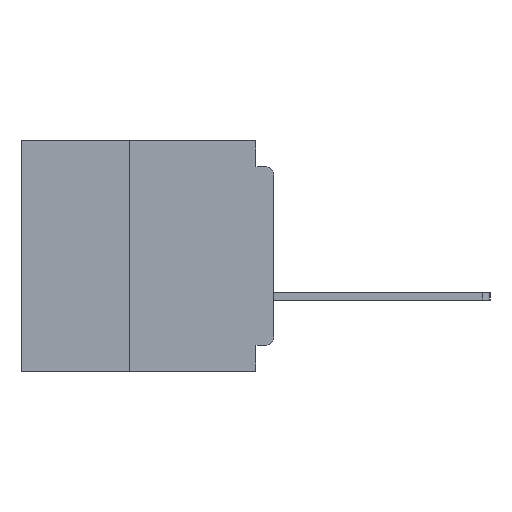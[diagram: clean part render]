
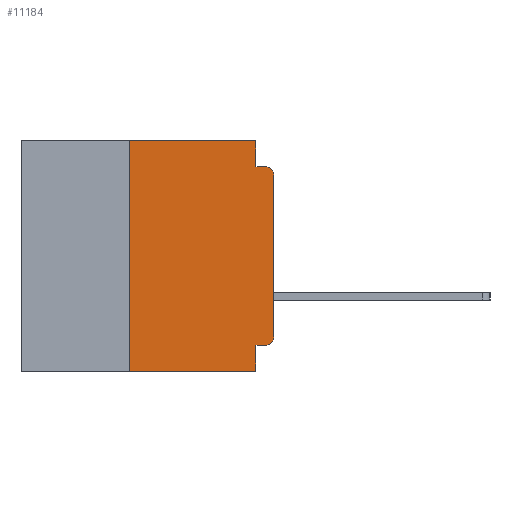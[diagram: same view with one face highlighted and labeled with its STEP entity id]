
A CAD part, left-side view. The second image highlights one B-rep face of the part: STEP entity #11184.
In plain terms, the highlighted planar face has unit normal (-1, 0, 0).
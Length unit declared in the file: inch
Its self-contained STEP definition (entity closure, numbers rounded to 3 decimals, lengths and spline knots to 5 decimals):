
#19 = VERTEX_POINT ( 'NONE', #27709 ) ;
#135 = DIRECTION ( 'NONE',  ( 0., 0., -1. ) ) ;
#626 = ORIENTED_EDGE ( 'NONE', *, *, #46272, .T. ) ;
#731 = EDGE_CURVE ( 'NONE', #19723, #12528, #26812, .T. ) ;
#824 = VERTEX_POINT ( 'NONE', #867 ) ;
#867 = CARTESIAN_POINT ( 'NONE',  ( 0., 0.015, -0.355 ) ) ;
#1844 = ORIENTED_EDGE ( 'NONE', *, *, #19192, .F. ) ;
#2385 = DIRECTION ( 'NONE',  ( 0., 0., 1. ) ) ;
#2674 = CARTESIAN_POINT ( 'NONE',  ( 0., 0.437, 0. ) ) ;
#3344 = VECTOR ( 'NONE', #25679, 39.37008 ) ;
#3861 = CARTESIAN_POINT ( 'NONE',  ( 0., 0.031, 0. ) ) ;
#3969 = ORIENTED_EDGE ( 'NONE', *, *, #53702, .F. ) ;
#4319 = LINE ( 'NONE', #39994, #36277 ) ;
#5255 = ORIENTED_EDGE ( 'NONE', *, *, #39785, .T. ) ;
#5553 = VECTOR ( 'NONE', #36344, 39.37008 ) ;
#6567 = VECTOR ( 'NONE', #48807, 39.37008 ) ;
#10461 = VECTOR ( 'NONE', #47812, 39.37008 ) ;
#10559 = FACE_OUTER_BOUND ( 'NONE', #38248, .T. ) ;
#11108 = DIRECTION ( 'NONE',  ( 0., 0., -1. ) ) ;
#11184 = ADVANCED_FACE ( 'NONE', ( #10559 ), #27646, .F. ) ;
#11774 = LINE ( 'NONE', #43641, #10461 ) ;
#12528 = VERTEX_POINT ( 'NONE', #16664 ) ;
#13629 = CIRCLE ( 'NONE', #18632, 0.015 ) ;
#13636 = CARTESIAN_POINT ( 'NONE',  ( 0., 0.031, -0.045 ) ) ;
#13940 = DIRECTION ( 'NONE',  ( -1., 0., 0. ) ) ;
#14809 = EDGE_CURVE ( 'NONE', #824, #19, #47758, .T. ) ;
#14965 = LINE ( 'NONE', #25106, #27288 ) ;
#15482 = CARTESIAN_POINT ( 'NONE',  ( 0., 0.437, -0.4 ) ) ;
#16664 = CARTESIAN_POINT ( 'NONE',  ( 0., 0.015, -0.045 ) ) ;
#17048 = ORIENTED_EDGE ( 'NONE', *, *, #33296, .F. ) ;
#17088 = VECTOR ( 'NONE', #29060, 39.37008 ) ;
#17284 = CARTESIAN_POINT ( 'NONE',  ( 0., 0.25, 0. ) ) ;
#17345 = AXIS2_PLACEMENT_3D ( 'NONE', #2674, #36056, #11108 ) ;
#17492 = LINE ( 'NONE', #37198, #38333 ) ;
#18632 = AXIS2_PLACEMENT_3D ( 'NONE', #38877, #13940, #43110 ) ;
#19192 = EDGE_CURVE ( 'NONE', #30142, #20017, #14965, .T. ) ;
#19723 = VERTEX_POINT ( 'NONE', #24155 ) ;
#20017 = VERTEX_POINT ( 'NONE', #13636 ) ;
#22823 = ORIENTED_EDGE ( 'NONE', *, *, #731, .T. ) ;
#23717 = CARTESIAN_POINT ( 'NONE',  ( 0., 0., 0. ) ) ;
#24155 = CARTESIAN_POINT ( 'NONE',  ( 0., 0., -0.06 ) ) ;
#24227 = DIRECTION ( 'NONE',  ( 0., 0., -1. ) ) ;
#24740 = DIRECTION ( 'NONE',  ( 0., -1., 0. ) ) ;
#25106 = CARTESIAN_POINT ( 'NONE',  ( 0., 0.031, 0. ) ) ;
#25481 = LINE ( 'NONE', #53989, #17088 ) ;
#25487 = ORIENTED_EDGE ( 'NONE', *, *, #44854, .T. ) ;
#25679 = DIRECTION ( 'NONE',  ( 0., 1., 0. ) ) ;
#26812 = CIRCLE ( 'NONE', #31151, 0.015 ) ;
#27288 = VECTOR ( 'NONE', #135, 39.37008 ) ;
#27646 = PLANE ( 'NONE',  #17345 ) ;
#27709 = CARTESIAN_POINT ( 'NONE',  ( 0., 0.031, -0.355 ) ) ;
#28604 = EDGE_CURVE ( 'NONE', #19, #39397, #11774, .T. ) ;
#28773 = LINE ( 'NONE', #15482, #6567 ) ;
#28944 = CARTESIAN_POINT ( 'NONE',  ( 0., 0.015, -0.06 ) ) ;
#29060 = DIRECTION ( 'NONE',  ( 0., -1., 0. ) ) ;
#29624 = VERTEX_POINT ( 'NONE', #17284 ) ;
#29932 = CARTESIAN_POINT ( 'NONE',  ( 0., 0., -0.355 ) ) ;
#30142 = VERTEX_POINT ( 'NONE', #3861 ) ;
#31151 = AXIS2_PLACEMENT_3D ( 'NONE', #28944, #34149, #24227 ) ;
#32635 = CARTESIAN_POINT ( 'NONE',  ( 0., 0., -0.34 ) ) ;
#33296 = EDGE_CURVE ( 'NONE', #20017, #12528, #25481, .T. ) ;
#33319 = ORIENTED_EDGE ( 'NONE', *, *, #45220, .F. ) ;
#34149 = DIRECTION ( 'NONE',  ( -1., 0., 0. ) ) ;
#36056 = DIRECTION ( 'NONE',  ( 1., 0., 0. ) ) ;
#36277 = VECTOR ( 'NONE', #2385, 39.37008 ) ;
#36344 = DIRECTION ( 'NONE',  ( 0., 0., 1. ) ) ;
#37198 = CARTESIAN_POINT ( 'NONE',  ( 0., 0.437, 0. ) ) ;
#38161 = CARTESIAN_POINT ( 'NONE',  ( 0., 0.25, -0.4 ) ) ;
#38248 = EDGE_LOOP ( 'NONE', ( #626, #22823, #17048, #1844, #33319, #3969, #5255, #41217, #42534, #25487 ) ) ;
#38333 = VECTOR ( 'NONE', #24740, 39.37008 ) ;
#38877 = CARTESIAN_POINT ( 'NONE',  ( 0., 0.015, -0.34 ) ) ;
#39397 = VERTEX_POINT ( 'NONE', #50464 ) ;
#39785 = EDGE_CURVE ( 'NONE', #44751, #39397, #28773, .T. ) ;
#39994 = CARTESIAN_POINT ( 'NONE',  ( 0., 0.25, -0.4 ) ) ;
#41217 = ORIENTED_EDGE ( 'NONE', *, *, #28604, .F. ) ;
#42534 = ORIENTED_EDGE ( 'NONE', *, *, #14809, .F. ) ;
#42936 = VERTEX_POINT ( 'NONE', #32635 ) ;
#43110 = DIRECTION ( 'NONE',  ( 0., 0., -1. ) ) ;
#43641 = CARTESIAN_POINT ( 'NONE',  ( 0., 0.031, -0.4 ) ) ;
#44751 = VERTEX_POINT ( 'NONE', #38161 ) ;
#44854 = EDGE_CURVE ( 'NONE', #824, #42936, #13629, .T. ) ;
#45220 = EDGE_CURVE ( 'NONE', #29624, #30142, #17492, .T. ) ;
#46272 = EDGE_CURVE ( 'NONE', #42936, #19723, #49938, .T. ) ;
#47758 = LINE ( 'NONE', #29932, #3344 ) ;
#47812 = DIRECTION ( 'NONE',  ( 0., 0., -1. ) ) ;
#48807 = DIRECTION ( 'NONE',  ( 0., -1., 0. ) ) ;
#49938 = LINE ( 'NONE', #23717, #5553 ) ;
#50464 = CARTESIAN_POINT ( 'NONE',  ( 0., 0.031, -0.4 ) ) ;
#53702 = EDGE_CURVE ( 'NONE', #44751, #29624, #4319, .T. ) ;
#53989 = CARTESIAN_POINT ( 'NONE',  ( 0., 0., -0.045 ) ) ;
